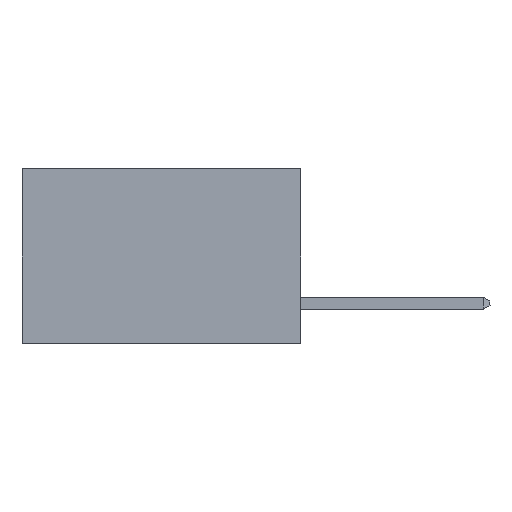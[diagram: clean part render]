
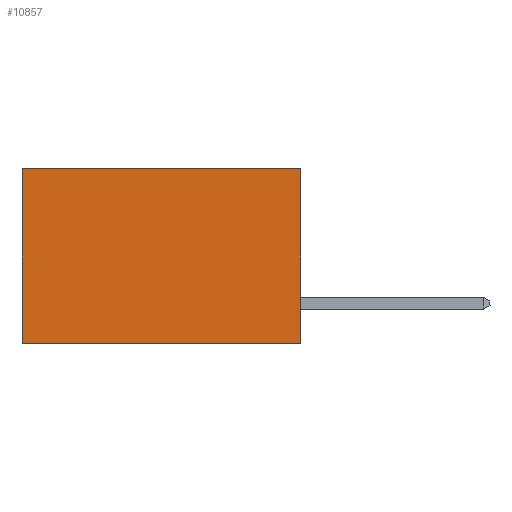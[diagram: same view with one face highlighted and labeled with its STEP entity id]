
A CAD part, left-side view. The second image highlights one B-rep face of the part: STEP entity #10857.
In plain terms, the highlighted planar face has unit normal (-1, 0, 0).
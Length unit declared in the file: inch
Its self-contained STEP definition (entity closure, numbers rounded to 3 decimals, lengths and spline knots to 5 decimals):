
#600 = CARTESIAN_POINT ( 'NONE',  ( 0.277, 0., -0.37 ) ) ;
#658 = DIRECTION ( 'NONE',  ( 0., 0., -1. ) ) ;
#792 = CARTESIAN_POINT ( 'NONE',  ( 0.277, 0.59, -0.37 ) ) ;
#1290 = VECTOR ( 'NONE', #4277, 39.37008 ) ;
#1304 = EDGE_CURVE ( 'NONE', #11273, #10807, #7413, .T. ) ;
#1749 = LINE ( 'NONE', #8020, #6687 ) ;
#1897 = EDGE_LOOP ( 'NONE', ( #3471, #8896, #11450, #3802 ) ) ;
#3471 = ORIENTED_EDGE ( 'NONE', *, *, #1304, .T. ) ;
#3537 = CARTESIAN_POINT ( 'NONE',  ( 0.277, 0., 0. ) ) ;
#3802 = ORIENTED_EDGE ( 'NONE', *, *, #9694, .T. ) ;
#3820 = LINE ( 'NONE', #600, #11466 ) ;
#4199 = CARTESIAN_POINT ( 'NONE',  ( 0.277, 0., -0.37 ) ) ;
#4277 = DIRECTION ( 'NONE',  ( 0., 1., 0. ) ) ;
#5241 = CARTESIAN_POINT ( 'NONE',  ( 0.277, 0., -0.37 ) ) ;
#5260 = DIRECTION ( 'NONE',  ( 0., 0., -1. ) ) ;
#5573 = AXIS2_PLACEMENT_3D ( 'NONE', #4199, #11160, #5260 ) ;
#6124 = EDGE_CURVE ( 'NONE', #11930, #11610, #3820, .T. ) ;
#6257 = PLANE ( 'NONE',  #5573 ) ;
#6687 = VECTOR ( 'NONE', #9021, 39.37008 ) ;
#6705 = EDGE_CURVE ( 'NONE', #11610, #10807, #9521, .T. ) ;
#7413 = LINE ( 'NONE', #12379, #12240 ) ;
#8020 = CARTESIAN_POINT ( 'NONE',  ( 0.277, 0., 0. ) ) ;
#8896 = ORIENTED_EDGE ( 'NONE', *, *, #6705, .F. ) ;
#9021 = DIRECTION ( 'NONE',  ( 0., 1., 0. ) ) ;
#9521 = LINE ( 'NONE', #10282, #1290 ) ;
#9694 = EDGE_CURVE ( 'NONE', #11930, #11273, #1749, .T. ) ;
#10282 = CARTESIAN_POINT ( 'NONE',  ( 0.277, 0., -0.37 ) ) ;
#10807 = VERTEX_POINT ( 'NONE', #792 ) ;
#10857 = ADVANCED_FACE ( 'NONE', ( #11973 ), #6257, .F. ) ;
#11160 = DIRECTION ( 'NONE',  ( 1., 0., 0. ) ) ;
#11273 = VERTEX_POINT ( 'NONE', #12635 ) ;
#11450 = ORIENTED_EDGE ( 'NONE', *, *, #6124, .F. ) ;
#11466 = VECTOR ( 'NONE', #658, 39.37008 ) ;
#11610 = VERTEX_POINT ( 'NONE', #5241 ) ;
#11930 = VERTEX_POINT ( 'NONE', #3537 ) ;
#11973 = FACE_OUTER_BOUND ( 'NONE', #1897, .T. ) ;
#12240 = VECTOR ( 'NONE', #12294, 39.37008 ) ;
#12294 = DIRECTION ( 'NONE',  ( 0., 0., -1. ) ) ;
#12379 = CARTESIAN_POINT ( 'NONE',  ( 0.277, 0.59, -0.37 ) ) ;
#12635 = CARTESIAN_POINT ( 'NONE',  ( 0.277, 0.59, 0. ) ) ;
